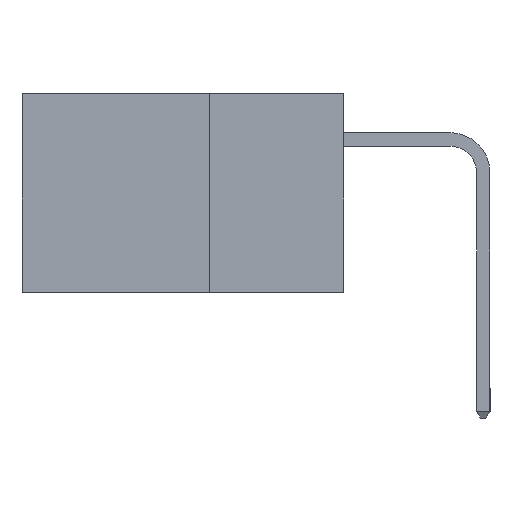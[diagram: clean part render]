
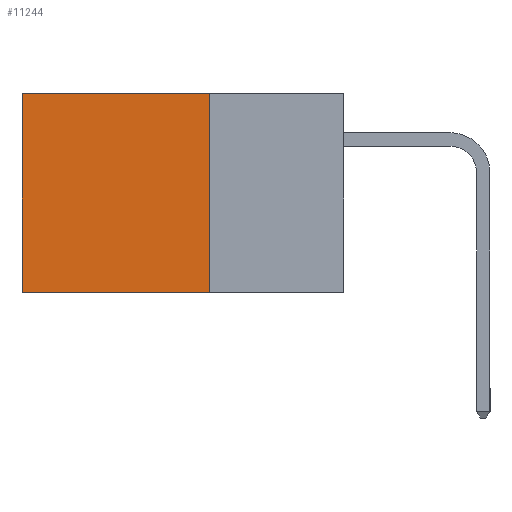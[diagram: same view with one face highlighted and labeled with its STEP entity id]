
A CAD part, left-side view. The second image highlights one B-rep face of the part: STEP entity #11244.
In plain terms, the highlighted planar face has unit normal (-1, 0, 0).
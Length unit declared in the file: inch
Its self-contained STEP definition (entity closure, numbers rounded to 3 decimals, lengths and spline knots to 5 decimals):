
#144 = VECTOR ( 'NONE', #9027, 39.37008 ) ;
#969 = EDGE_CURVE ( 'NONE', #11186, #10826, #13466, .T. ) ;
#1162 = EDGE_CURVE ( 'NONE', #13327, #4204, #18083, .T. ) ;
#2302 = ORIENTED_EDGE ( 'NONE', *, *, #1162, .T. ) ;
#2797 = VECTOR ( 'NONE', #4439, 39.37008 ) ;
#3645 = VECTOR ( 'NONE', #6348, 39.37008 ) ;
#4204 = VERTEX_POINT ( 'NONE', #19061 ) ;
#4439 = DIRECTION ( 'NONE',  ( 0., 0., -1. ) ) ;
#4723 = LINE ( 'NONE', #6287, #3645 ) ;
#6083 = CARTESIAN_POINT ( 'NONE',  ( 0.298, 0.25, -0.37 ) ) ;
#6287 = CARTESIAN_POINT ( 'NONE',  ( 0.298, 0.25, 0. ) ) ;
#6304 = DIRECTION ( 'NONE',  ( 1., 0., 0. ) ) ;
#6348 = DIRECTION ( 'NONE',  ( 0., 0., -1. ) ) ;
#6517 = EDGE_CURVE ( 'NONE', #13327, #11186, #4723, .T. ) ;
#7531 = FACE_OUTER_BOUND ( 'NONE', #8378, .T. ) ;
#8378 = EDGE_LOOP ( 'NONE', ( #19392, #14347, #11670, #2302 ) ) ;
#9027 = DIRECTION ( 'NONE',  ( 0., 1., 0. ) ) ;
#9905 = EDGE_CURVE ( 'NONE', #4204, #10826, #16663, .T. ) ;
#10826 = VERTEX_POINT ( 'NONE', #13552 ) ;
#11158 = CARTESIAN_POINT ( 'NONE',  ( 0.298, 0.6, 0. ) ) ;
#11186 = VERTEX_POINT ( 'NONE', #6083 ) ;
#11244 = ADVANCED_FACE ( 'NONE', ( #7531 ), #14624, .F. ) ;
#11670 = ORIENTED_EDGE ( 'NONE', *, *, #6517, .F. ) ;
#13327 = VERTEX_POINT ( 'NONE', #18867 ) ;
#13466 = LINE ( 'NONE', #18221, #144 ) ;
#13552 = CARTESIAN_POINT ( 'NONE',  ( 0.298, 0.6, -0.37 ) ) ;
#13726 = VECTOR ( 'NONE', #20639, 39.37008 ) ;
#14347 = ORIENTED_EDGE ( 'NONE', *, *, #969, .F. ) ;
#14624 = PLANE ( 'NONE',  #19633 ) ;
#16275 = CARTESIAN_POINT ( 'NONE',  ( 0.298, 0.25, 0. ) ) ;
#16663 = LINE ( 'NONE', #11158, #2797 ) ;
#17912 = DIRECTION ( 'NONE',  ( 0., 0., -1. ) ) ;
#18083 = LINE ( 'NONE', #20821, #13726 ) ;
#18221 = CARTESIAN_POINT ( 'NONE',  ( 0.298, 0.25, -0.37 ) ) ;
#18867 = CARTESIAN_POINT ( 'NONE',  ( 0.298, 0.25, 0. ) ) ;
#19061 = CARTESIAN_POINT ( 'NONE',  ( 0.298, 0.6, 0. ) ) ;
#19392 = ORIENTED_EDGE ( 'NONE', *, *, #9905, .T. ) ;
#19633 = AXIS2_PLACEMENT_3D ( 'NONE', #16275, #6304, #17912 ) ;
#20639 = DIRECTION ( 'NONE',  ( 0., 1., 0. ) ) ;
#20821 = CARTESIAN_POINT ( 'NONE',  ( 0.298, 0.25, 0. ) ) ;
